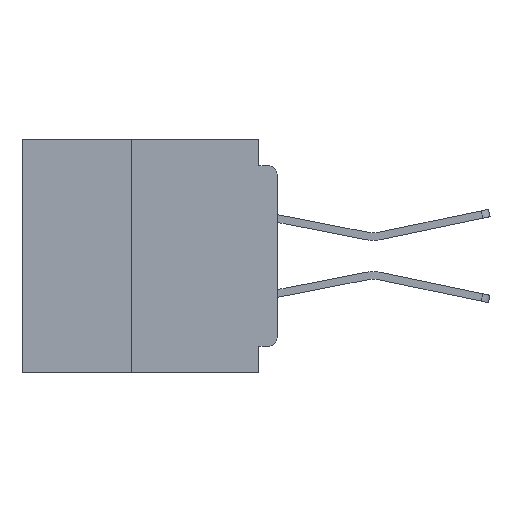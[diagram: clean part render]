
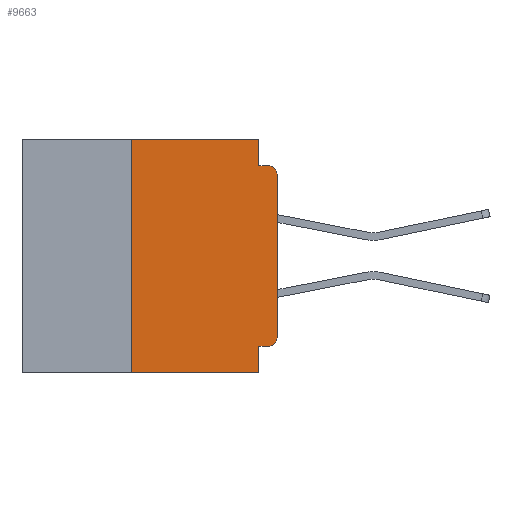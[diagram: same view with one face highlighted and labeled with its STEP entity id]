
A CAD part, left-side view. The second image highlights one B-rep face of the part: STEP entity #9663.
In plain terms, the highlighted planar face has unit normal (-1, 0, 0).
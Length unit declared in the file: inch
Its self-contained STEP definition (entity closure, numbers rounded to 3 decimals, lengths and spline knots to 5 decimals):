
#451 = ORIENTED_EDGE ( 'NONE', *, *, #55330, .F. ) ;
#483 = CARTESIAN_POINT ( 'NONE',  ( 0., 0.015, -0.355 ) ) ;
#975 = VECTOR ( 'NONE', #26187, 39.37008 ) ;
#2562 = VECTOR ( 'NONE', #10094, 39.37008 ) ;
#2581 = DIRECTION ( 'NONE',  ( 0., 0., -1. ) ) ;
#3060 = CARTESIAN_POINT ( 'NONE',  ( 0., 0.25, 0. ) ) ;
#3431 = VECTOR ( 'NONE', #35462, 39.37008 ) ;
#3562 = CARTESIAN_POINT ( 'NONE',  ( 0., 0.015, -0.34 ) ) ;
#5999 = DIRECTION ( 'NONE',  ( 0., 0., -1. ) ) ;
#6127 = VERTEX_POINT ( 'NONE', #10489 ) ;
#6432 = EDGE_CURVE ( 'NONE', #37923, #32734, #40928, .T. ) ;
#7222 = EDGE_CURVE ( 'NONE', #52894, #20418, #34691, .T. ) ;
#7365 = DIRECTION ( 'NONE',  ( 0., 0., -1. ) ) ;
#7473 = DIRECTION ( 'NONE',  ( 0., 0., 1. ) ) ;
#7646 = ORIENTED_EDGE ( 'NONE', *, *, #8378, .F. ) ;
#7995 = DIRECTION ( 'NONE',  ( 0., 0., -1. ) ) ;
#8378 = EDGE_CURVE ( 'NONE', #25040, #52894, #17453, .T. ) ;
#9484 = LINE ( 'NONE', #12203, #43131 ) ;
#9663 = ADVANCED_FACE ( 'NONE', ( #22818 ), #20106, .F. ) ;
#10094 = DIRECTION ( 'NONE',  ( 0., 0., 1. ) ) ;
#10443 = CARTESIAN_POINT ( 'NONE',  ( 0., 0.25, -0.4 ) ) ;
#10489 = CARTESIAN_POINT ( 'NONE',  ( 0., 0., -0.06 ) ) ;
#12203 = CARTESIAN_POINT ( 'NONE',  ( 0., 0.437, 0. ) ) ;
#13092 = ORIENTED_EDGE ( 'NONE', *, *, #13398, .F. ) ;
#13226 = ORIENTED_EDGE ( 'NONE', *, *, #34887, .T. ) ;
#13398 = EDGE_CURVE ( 'NONE', #37923, #22809, #35557, .T. ) ;
#13538 = CARTESIAN_POINT ( 'NONE',  ( 0., 0.015, -0.06 ) ) ;
#13706 = VECTOR ( 'NONE', #7365, 39.37008 ) ;
#14274 = LINE ( 'NONE', #40811, #2562 ) ;
#14642 = VERTEX_POINT ( 'NONE', #43249 ) ;
#15019 = CARTESIAN_POINT ( 'NONE',  ( 0., 0.031, 0. ) ) ;
#15116 = LINE ( 'NONE', #22243, #3431 ) ;
#15192 = VERTEX_POINT ( 'NONE', #3060 ) ;
#16022 = EDGE_LOOP ( 'NONE', ( #42829, #17691, #40209, #7646, #31747, #24708, #13226, #451, #13092, #51468 ) ) ;
#16866 = CARTESIAN_POINT ( 'NONE',  ( 0., 0., -0.355 ) ) ;
#17453 = LINE ( 'NONE', #15019, #40779 ) ;
#17691 = ORIENTED_EDGE ( 'NONE', *, *, #31113, .T. ) ;
#17991 = DIRECTION ( 'NONE',  ( 0., 0., -1. ) ) ;
#18801 = VERTEX_POINT ( 'NONE', #10443 ) ;
#20036 = AXIS2_PLACEMENT_3D ( 'NONE', #3562, #34312, #7995 ) ;
#20106 = PLANE ( 'NONE',  #43277 ) ;
#20418 = VERTEX_POINT ( 'NONE', #26892 ) ;
#21763 = CARTESIAN_POINT ( 'NONE',  ( 0., 0.031, -0.045 ) ) ;
#22243 = CARTESIAN_POINT ( 'NONE',  ( 0., 0.437, -0.4 ) ) ;
#22809 = VERTEX_POINT ( 'NONE', #23239 ) ;
#22818 = FACE_OUTER_BOUND ( 'NONE', #16022, .T. ) ;
#23239 = CARTESIAN_POINT ( 'NONE',  ( 0., 0.031, -0.355 ) ) ;
#24708 = ORIENTED_EDGE ( 'NONE', *, *, #29014, .F. ) ;
#25040 = VERTEX_POINT ( 'NONE', #41970 ) ;
#25328 = DIRECTION ( 'NONE',  ( 0., -1., 0. ) ) ;
#26187 = DIRECTION ( 'NONE',  ( 0., -1., 0. ) ) ;
#26892 = CARTESIAN_POINT ( 'NONE',  ( 0., 0.015, -0.045 ) ) ;
#27947 = VECTOR ( 'NONE', #7473, 39.37008 ) ;
#28757 = CARTESIAN_POINT ( 'NONE',  ( 0., 0.437, 0. ) ) ;
#28941 = DIRECTION ( 'NONE',  ( 1., 0., 0. ) ) ;
#29014 = EDGE_CURVE ( 'NONE', #18801, #15192, #51155, .T. ) ;
#29261 = CARTESIAN_POINT ( 'NONE',  ( 0., 0.031, -0.4 ) ) ;
#31113 = EDGE_CURVE ( 'NONE', #6127, #20418, #47703, .T. ) ;
#31747 = ORIENTED_EDGE ( 'NONE', *, *, #52147, .F. ) ;
#32734 = VERTEX_POINT ( 'NONE', #50632 ) ;
#34312 = DIRECTION ( 'NONE',  ( -1., 0., 0. ) ) ;
#34691 = LINE ( 'NONE', #48139, #975 ) ;
#34887 = EDGE_CURVE ( 'NONE', #18801, #14642, #15116, .T. ) ;
#35462 = DIRECTION ( 'NONE',  ( 0., -1., 0. ) ) ;
#35557 = LINE ( 'NONE', #16866, #47178 ) ;
#37923 = VERTEX_POINT ( 'NONE', #483 ) ;
#38754 = DIRECTION ( 'NONE',  ( 0., 1., 0. ) ) ;
#40209 = ORIENTED_EDGE ( 'NONE', *, *, #7222, .F. ) ;
#40779 = VECTOR ( 'NONE', #5999, 39.37008 ) ;
#40811 = CARTESIAN_POINT ( 'NONE',  ( 0., 0., 0. ) ) ;
#40928 = CIRCLE ( 'NONE', #20036, 0.015 ) ;
#41970 = CARTESIAN_POINT ( 'NONE',  ( 0., 0.031, 0. ) ) ;
#42829 = ORIENTED_EDGE ( 'NONE', *, *, #56325, .T. ) ;
#43131 = VECTOR ( 'NONE', #25328, 39.37008 ) ;
#43249 = CARTESIAN_POINT ( 'NONE',  ( 0., 0.031, -0.4 ) ) ;
#43277 = AXIS2_PLACEMENT_3D ( 'NONE', #28757, #28941, #2581 ) ;
#44231 = DIRECTION ( 'NONE',  ( -1., 0., 0. ) ) ;
#46945 = CARTESIAN_POINT ( 'NONE',  ( 0., 0.25, -0.4 ) ) ;
#47178 = VECTOR ( 'NONE', #38754, 39.37008 ) ;
#47703 = CIRCLE ( 'NONE', #49786, 0.015 ) ;
#48139 = CARTESIAN_POINT ( 'NONE',  ( 0., 0., -0.045 ) ) ;
#48669 = LINE ( 'NONE', #29261, #13706 ) ;
#49786 = AXIS2_PLACEMENT_3D ( 'NONE', #13538, #44231, #17991 ) ;
#50632 = CARTESIAN_POINT ( 'NONE',  ( 0., 0., -0.34 ) ) ;
#51155 = LINE ( 'NONE', #46945, #27947 ) ;
#51468 = ORIENTED_EDGE ( 'NONE', *, *, #6432, .T. ) ;
#52147 = EDGE_CURVE ( 'NONE', #15192, #25040, #9484, .T. ) ;
#52894 = VERTEX_POINT ( 'NONE', #21763 ) ;
#55330 = EDGE_CURVE ( 'NONE', #22809, #14642, #48669, .T. ) ;
#56325 = EDGE_CURVE ( 'NONE', #32734, #6127, #14274, .T. ) ;
